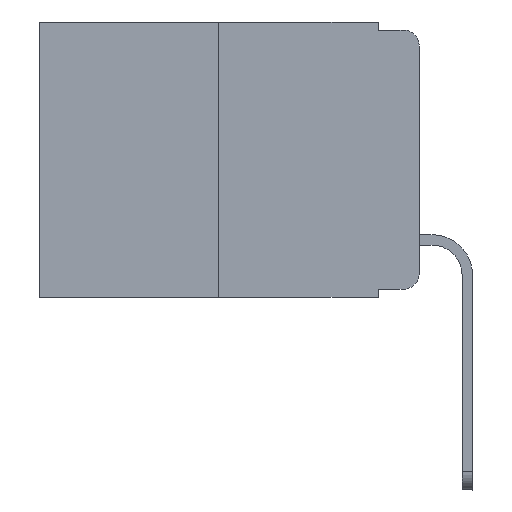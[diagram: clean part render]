
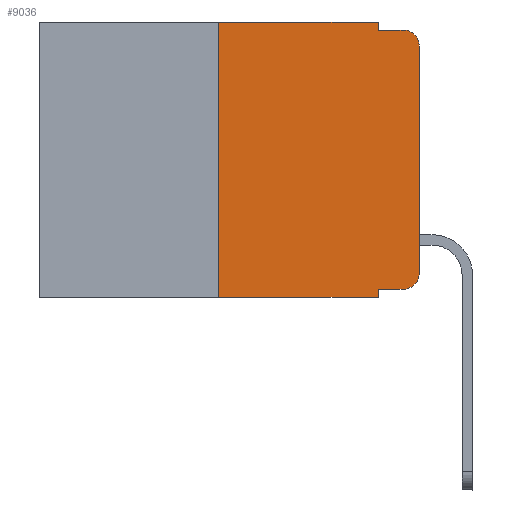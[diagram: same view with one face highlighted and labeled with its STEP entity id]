
A CAD part, left-side view. The second image highlights one B-rep face of the part: STEP entity #9036.
In plain terms, the highlighted planar face has unit normal (-1, 0, 0).
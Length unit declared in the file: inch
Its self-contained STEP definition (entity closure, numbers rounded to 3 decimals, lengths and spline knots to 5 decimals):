
#52 = LINE ( 'NONE', #1968, #14874 ) ;
#914 = VERTEX_POINT ( 'NONE', #3321 ) ;
#1167 = AXIS2_PLACEMENT_3D ( 'NONE', #5418, #18994, #23195 ) ;
#1197 = CARTESIAN_POINT ( 'NONE',  ( 0., 0.473, -0.343 ) ) ;
#1824 = EDGE_CURVE ( 'NONE', #14981, #9758, #52, .T. ) ;
#1968 = CARTESIAN_POINT ( 'NONE',  ( 0., 0.051, -0.333 ) ) ;
#2098 = VERTEX_POINT ( 'NONE', #7135 ) ;
#2594 = AXIS2_PLACEMENT_3D ( 'NONE', #12511, #16325, #13892 ) ;
#2737 = VERTEX_POINT ( 'NONE', #7471 ) ;
#2957 = LINE ( 'NONE', #1197, #14357 ) ;
#3321 = CARTESIAN_POINT ( 'NONE',  ( 0., 0., -0.313 ) ) ;
#3524 = EDGE_CURVE ( 'NONE', #9758, #914, #21229, .T. ) ;
#4226 = CARTESIAN_POINT ( 'NONE',  ( 0., 0.051, 0. ) ) ;
#4379 = VECTOR ( 'NONE', #23033, 39.37008 ) ;
#4698 = ORIENTED_EDGE ( 'NONE', *, *, #14506, .T. ) ;
#4926 = DIRECTION ( 'NONE',  ( 0., -1., 0. ) ) ;
#5418 = CARTESIAN_POINT ( 'NONE',  ( 0., 0.473, 0. ) ) ;
#6255 = EDGE_LOOP ( 'NONE', ( #23184, #4698, #11280, #15719, #23806, #20694, #8211, #10258, #13034, #19829 ) ) ;
#6482 = VERTEX_POINT ( 'NONE', #22399 ) ;
#6754 = EDGE_CURVE ( 'NONE', #2737, #20156, #18312, .T. ) ;
#7096 = VECTOR ( 'NONE', #15929, 39.37008 ) ;
#7135 = CARTESIAN_POINT ( 'NONE',  ( 0., 0.25, -0.343 ) ) ;
#7471 = CARTESIAN_POINT ( 'NONE',  ( 0., 0.051, 0. ) ) ;
#7564 = FACE_OUTER_BOUND ( 'NONE', #6255, .T. ) ;
#7685 = PLANE ( 'NONE',  #1167 ) ;
#7855 = CARTESIAN_POINT ( 'NONE',  ( 0., 0., -0.03 ) ) ;
#8147 = EDGE_CURVE ( 'NONE', #914, #14490, #9413, .T. ) ;
#8211 = ORIENTED_EDGE ( 'NONE', *, *, #21879, .T. ) ;
#8365 = DIRECTION ( 'NONE',  ( 0., 0., -1. ) ) ;
#8396 = DIRECTION ( 'NONE',  ( 0., 0., -1. ) ) ;
#8709 = LINE ( 'NONE', #18489, #15096 ) ;
#8923 = DIRECTION ( 'NONE',  ( 0., -1., 0. ) ) ;
#9036 = ADVANCED_FACE ( 'NONE', ( #7564 ), #7685, .F. ) ;
#9413 = LINE ( 'NONE', #9677, #4379 ) ;
#9677 = CARTESIAN_POINT ( 'NONE',  ( 0., 0., 0. ) ) ;
#9758 = VERTEX_POINT ( 'NONE', #14492 ) ;
#9980 = CARTESIAN_POINT ( 'NONE',  ( 0., 0.051, -0.333 ) ) ;
#10257 = DIRECTION ( 'NONE',  ( -1., 0., 0. ) ) ;
#10258 = ORIENTED_EDGE ( 'NONE', *, *, #20138, .F. ) ;
#10611 = VERTEX_POINT ( 'NONE', #14907 ) ;
#11280 = ORIENTED_EDGE ( 'NONE', *, *, #19346, .F. ) ;
#12113 = CARTESIAN_POINT ( 'NONE',  ( 0., 0.25, 0. ) ) ;
#12511 = CARTESIAN_POINT ( 'NONE',  ( 0., 0.02, -0.313 ) ) ;
#13034 = ORIENTED_EDGE ( 'NONE', *, *, #1824, .T. ) ;
#13658 = CARTESIAN_POINT ( 'NONE',  ( 0., 0.051, -0.01 ) ) ;
#13892 = DIRECTION ( 'NONE',  ( 0., 0., -1. ) ) ;
#14357 = VECTOR ( 'NONE', #24418, 39.37008 ) ;
#14490 = VERTEX_POINT ( 'NONE', #7855 ) ;
#14492 = CARTESIAN_POINT ( 'NONE',  ( 0., 0.02, -0.333 ) ) ;
#14506 = EDGE_CURVE ( 'NONE', #14490, #15389, #20385, .T. ) ;
#14513 = CARTESIAN_POINT ( 'NONE',  ( 0., 0.051, -0.01 ) ) ;
#14874 = VECTOR ( 'NONE', #23043, 39.37008 ) ;
#14907 = CARTESIAN_POINT ( 'NONE',  ( 0., 0.25, 0. ) ) ;
#14981 = VERTEX_POINT ( 'NONE', #9980 ) ;
#15096 = VECTOR ( 'NONE', #4926, 39.37008 ) ;
#15389 = VERTEX_POINT ( 'NONE', #17935 ) ;
#15667 = LINE ( 'NONE', #12113, #7096 ) ;
#15719 = ORIENTED_EDGE ( 'NONE', *, *, #6754, .F. ) ;
#15929 = DIRECTION ( 'NONE',  ( 0., 0., 1. ) ) ;
#16325 = DIRECTION ( 'NONE',  ( -1., 0., 0. ) ) ;
#17098 = CARTESIAN_POINT ( 'NONE',  ( 0., 0.051, 0. ) ) ;
#17935 = CARTESIAN_POINT ( 'NONE',  ( 0., 0.02, -0.01 ) ) ;
#18312 = LINE ( 'NONE', #4226, #23127 ) ;
#18489 = CARTESIAN_POINT ( 'NONE',  ( 0., 0.473, 0. ) ) ;
#18933 = EDGE_CURVE ( 'NONE', #10611, #2737, #8709, .T. ) ;
#18994 = DIRECTION ( 'NONE',  ( 1., 0., 0. ) ) ;
#19002 = LINE ( 'NONE', #17098, #24879 ) ;
#19177 = VECTOR ( 'NONE', #8923, 39.37008 ) ;
#19346 = EDGE_CURVE ( 'NONE', #20156, #15389, #20115, .T. ) ;
#19670 = CARTESIAN_POINT ( 'NONE',  ( 0., 0.02, -0.03 ) ) ;
#19829 = ORIENTED_EDGE ( 'NONE', *, *, #3524, .T. ) ;
#20115 = LINE ( 'NONE', #14513, #19177 ) ;
#20138 = EDGE_CURVE ( 'NONE', #14981, #6482, #19002, .T. ) ;
#20156 = VERTEX_POINT ( 'NONE', #13658 ) ;
#20385 = CIRCLE ( 'NONE', #21598, 0.02 ) ;
#20694 = ORIENTED_EDGE ( 'NONE', *, *, #23040, .F. ) ;
#21229 = CIRCLE ( 'NONE', #2594, 0.02 ) ;
#21598 = AXIS2_PLACEMENT_3D ( 'NONE', #19670, #10257, #8365 ) ;
#21879 = EDGE_CURVE ( 'NONE', #2098, #6482, #2957, .T. ) ;
#22399 = CARTESIAN_POINT ( 'NONE',  ( 0., 0.051, -0.343 ) ) ;
#23033 = DIRECTION ( 'NONE',  ( 0., 0., 1. ) ) ;
#23040 = EDGE_CURVE ( 'NONE', #2098, #10611, #15667, .T. ) ;
#23043 = DIRECTION ( 'NONE',  ( 0., -1., 0. ) ) ;
#23127 = VECTOR ( 'NONE', #8396, 39.37008 ) ;
#23184 = ORIENTED_EDGE ( 'NONE', *, *, #8147, .T. ) ;
#23195 = DIRECTION ( 'NONE',  ( 0., 0., -1. ) ) ;
#23806 = ORIENTED_EDGE ( 'NONE', *, *, #18933, .F. ) ;
#24418 = DIRECTION ( 'NONE',  ( 0., -1., 0. ) ) ;
#24849 = DIRECTION ( 'NONE',  ( 0., 0., -1. ) ) ;
#24879 = VECTOR ( 'NONE', #24849, 39.37008 ) ;
